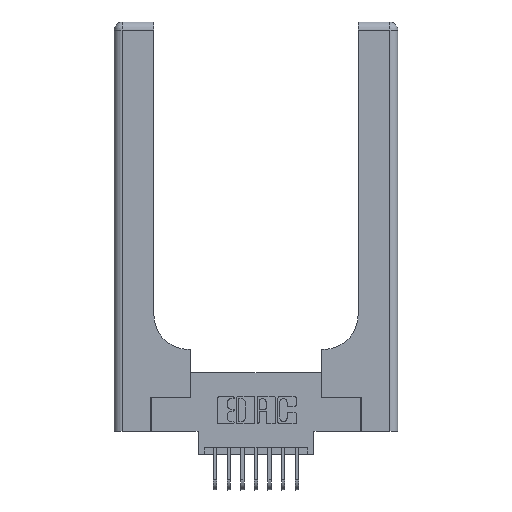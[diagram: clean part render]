
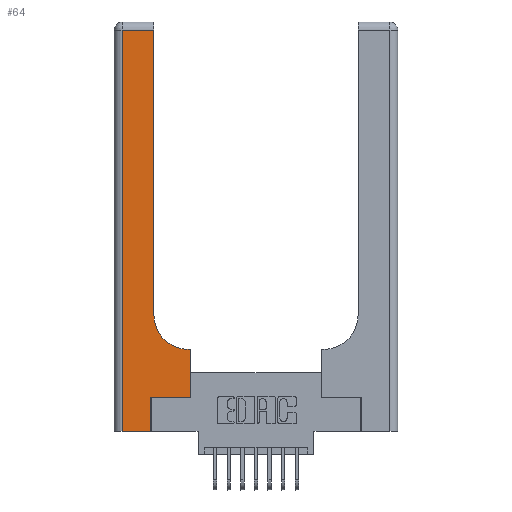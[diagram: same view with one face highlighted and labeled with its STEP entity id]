
A CAD part, top view. The second image highlights one B-rep face of the part: STEP entity #64.
In plain terms, the highlighted planar face has unit normal (0, 0, 1).
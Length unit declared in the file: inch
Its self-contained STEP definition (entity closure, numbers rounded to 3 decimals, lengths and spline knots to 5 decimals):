
#64 = ADVANCED_FACE ( 'NONE', ( #12626 ), #10825, .F. ) ;
#286 = ORIENTED_EDGE ( 'NONE', *, *, #3625, .T. ) ;
#519 = CARTESIAN_POINT ( 'NONE',  ( 0.269, 0.25, 0.37 ) ) ;
#1091 = EDGE_CURVE ( 'NONE', #9654, #12355, #1856, .T. ) ;
#1163 = CIRCLE ( 'NONE', #1515, 0.25 ) ;
#1211 = CARTESIAN_POINT ( 'NONE',  ( 0.2915, 2.94, 0.37 ) ) ;
#1515 = AXIS2_PLACEMENT_3D ( 'NONE', #9816, #1768, #11165 ) ;
#1768 = DIRECTION ( 'NONE',  ( 0., 0., -1. ) ) ;
#1856 = LINE ( 'NONE', #1963, #13023 ) ;
#1963 = CARTESIAN_POINT ( 'NONE',  ( 0., 2.94, 0.37 ) ) ;
#2468 = CARTESIAN_POINT ( 'NONE',  ( 0.2915, 3., 0.37 ) ) ;
#2568 = ORIENTED_EDGE ( 'NONE', *, *, #9344, .T. ) ;
#2710 = CARTESIAN_POINT ( 'NONE',  ( 0.269, 0.25, 0.37 ) ) ;
#3405 = VERTEX_POINT ( 'NONE', #519 ) ;
#3625 = EDGE_CURVE ( 'NONE', #9780, #15310, #1163, .T. ) ;
#3725 = EDGE_LOOP ( 'NONE', ( #8870, #15919, #16325, #2568, #9722, #16736, #6618, #7014, #286 ) ) ;
#3767 = LINE ( 'NONE', #8111, #10889 ) ;
#4335 = CARTESIAN_POINT ( 'NONE',  ( 0.269, 0., 0.37 ) ) ;
#5332 = CARTESIAN_POINT ( 'NONE',  ( 0.269, 0., 0.37 ) ) ;
#5642 = DIRECTION ( 'NONE',  ( -1., 0., 0. ) ) ;
#6389 = VECTOR ( 'NONE', #16051, 39.37008 ) ;
#6575 = DIRECTION ( 'NONE',  ( 0., 1., 0. ) ) ;
#6618 = ORIENTED_EDGE ( 'NONE', *, *, #11930, .T. ) ;
#6677 = VECTOR ( 'NONE', #12360, 39.37008 ) ;
#6900 = VERTEX_POINT ( 'NONE', #10526 ) ;
#6920 = EDGE_CURVE ( 'NONE', #15310, #9654, #12089, .T. ) ;
#6996 = VERTEX_POINT ( 'NONE', #5332 ) ;
#7014 = ORIENTED_EDGE ( 'NONE', *, *, #15147, .T. ) ;
#7131 = DIRECTION ( 'NONE',  ( 1., 0., 0. ) ) ;
#7585 = VECTOR ( 'NONE', #7131, 39.37008 ) ;
#8081 = VECTOR ( 'NONE', #6575, 39.37008 ) ;
#8102 = VERTEX_POINT ( 'NONE', #12188 ) ;
#8111 = CARTESIAN_POINT ( 'NONE',  ( 0.5585, 0.25, 0.37 ) ) ;
#8200 = DIRECTION ( 'NONE',  ( -1., 0., 0. ) ) ;
#8435 = CARTESIAN_POINT ( 'NONE',  ( 0.5415, 0.6, 0.37 ) ) ;
#8446 = VERTEX_POINT ( 'NONE', #15534 ) ;
#8558 = DIRECTION ( 'NONE',  ( 0., 0., -1. ) ) ;
#8735 = CARTESIAN_POINT ( 'NONE',  ( 0., 3., 0.37 ) ) ;
#8870 = ORIENTED_EDGE ( 'NONE', *, *, #6920, .T. ) ;
#9344 = EDGE_CURVE ( 'NONE', #8446, #6996, #14684, .T. ) ;
#9654 = VERTEX_POINT ( 'NONE', #1211 ) ;
#9722 = ORIENTED_EDGE ( 'NONE', *, *, #13702, .T. ) ;
#9780 = VERTEX_POINT ( 'NONE', #8435 ) ;
#9816 = CARTESIAN_POINT ( 'NONE',  ( 0.5415, 0.85, 0.37 ) ) ;
#10055 = CARTESIAN_POINT ( 'NONE',  ( 0.06, 3., 0.37 ) ) ;
#10207 = LINE ( 'NONE', #4335, #6677 ) ;
#10332 = LINE ( 'NONE', #2710, #6389 ) ;
#10526 = CARTESIAN_POINT ( 'NONE',  ( 0.5585, 0.6, 0.37 ) ) ;
#10825 = PLANE ( 'NONE',  #15346 ) ;
#10889 = VECTOR ( 'NONE', #16057, 39.37008 ) ;
#10982 = CARTESIAN_POINT ( 'NONE',  ( 0.2915, 0.6, 0.37 ) ) ;
#11165 = DIRECTION ( 'NONE',  ( 1., 0., 0. ) ) ;
#11812 = VECTOR ( 'NONE', #12349, 39.37008 ) ;
#11930 = EDGE_CURVE ( 'NONE', #8102, #6900, #3767, .T. ) ;
#12089 = LINE ( 'NONE', #2468, #8081 ) ;
#12188 = CARTESIAN_POINT ( 'NONE',  ( 0.5585, 0.25, 0.37 ) ) ;
#12226 = LINE ( 'NONE', #10982, #11812 ) ;
#12349 = DIRECTION ( 'NONE',  ( -1., 0., 0. ) ) ;
#12355 = VERTEX_POINT ( 'NONE', #15528 ) ;
#12360 = DIRECTION ( 'NONE',  ( 0., 1., 0. ) ) ;
#12626 = FACE_OUTER_BOUND ( 'NONE', #3725, .T. ) ;
#13023 = VECTOR ( 'NONE', #5642, 39.37008 ) ;
#13702 = EDGE_CURVE ( 'NONE', #6996, #3405, #10207, .T. ) ;
#14684 = LINE ( 'NONE', #16324, #7585 ) ;
#15055 = EDGE_CURVE ( 'NONE', #3405, #8102, #10332, .T. ) ;
#15147 = EDGE_CURVE ( 'NONE', #6900, #9780, #12226, .T. ) ;
#15192 = CARTESIAN_POINT ( 'NONE',  ( 0.2915, 0.85, 0.37 ) ) ;
#15310 = VERTEX_POINT ( 'NONE', #15192 ) ;
#15346 = AXIS2_PLACEMENT_3D ( 'NONE', #8735, #8558, #8200 ) ;
#15528 = CARTESIAN_POINT ( 'NONE',  ( 0.06, 2.94, 0.37 ) ) ;
#15534 = CARTESIAN_POINT ( 'NONE',  ( 0.06, 0., 0.37 ) ) ;
#15919 = ORIENTED_EDGE ( 'NONE', *, *, #1091, .T. ) ;
#16051 = DIRECTION ( 'NONE',  ( 1., 0., 0. ) ) ;
#16057 = DIRECTION ( 'NONE',  ( 0., 1., 0. ) ) ;
#16324 = CARTESIAN_POINT ( 'NONE',  ( 0., 0., 0.37 ) ) ;
#16325 = ORIENTED_EDGE ( 'NONE', *, *, #16532, .T. ) ;
#16464 = VECTOR ( 'NONE', #16631, 39.37008 ) ;
#16532 = EDGE_CURVE ( 'NONE', #12355, #8446, #16860, .T. ) ;
#16631 = DIRECTION ( 'NONE',  ( 0., -1., 0. ) ) ;
#16736 = ORIENTED_EDGE ( 'NONE', *, *, #15055, .T. ) ;
#16860 = LINE ( 'NONE', #10055, #16464 ) ;
